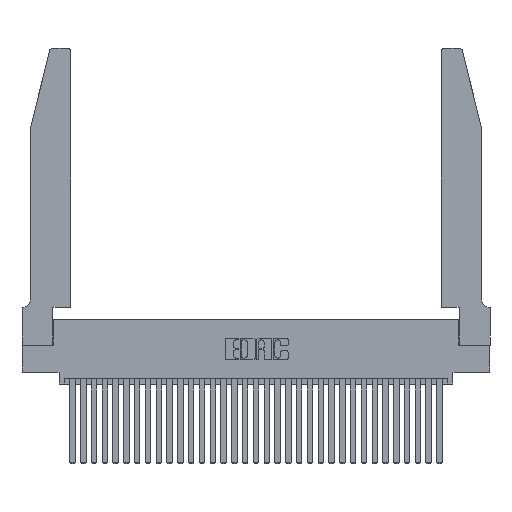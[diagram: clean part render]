
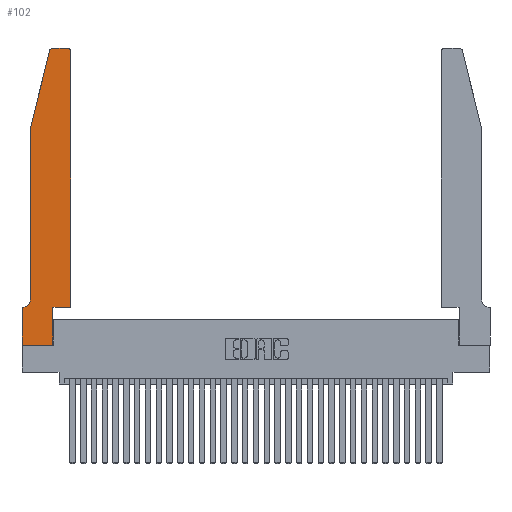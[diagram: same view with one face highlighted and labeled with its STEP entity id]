
A CAD part, top view. The second image highlights one B-rep face of the part: STEP entity #102.
In plain terms, the highlighted planar face has unit normal (0, 0, 1).
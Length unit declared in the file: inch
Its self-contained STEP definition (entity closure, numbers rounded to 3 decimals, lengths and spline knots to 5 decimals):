
#70 = CARTESIAN_POINT ( 'NONE',  ( 0., 0.35, 0.37 ) ) ;
#102 = ADVANCED_FACE ( 'NONE', ( #30458 ), #25693, .T. ) ;
#179 = CARTESIAN_POINT ( 'NONE',  ( 0.0755, 0.35, 0.37 ) ) ;
#722 = DIRECTION ( 'NONE',  ( 0., 0., 1. ) ) ;
#1178 = EDGE_CURVE ( 'NONE', #12635, #10571, #11612, .T. ) ;
#1284 = ORIENTED_EDGE ( 'NONE', *, *, #3603, .T. ) ;
#1601 = DIRECTION ( 'NONE',  ( 0., 0., 1. ) ) ;
#1818 = DIRECTION ( 'NONE',  ( 1., 0., 0. ) ) ;
#3047 = LINE ( 'NONE', #179, #16802 ) ;
#3603 = EDGE_CURVE ( 'NONE', #20287, #19433, #29973, .T. ) ;
#4251 = ORIENTED_EDGE ( 'NONE', *, *, #29277, .T. ) ;
#4355 = CARTESIAN_POINT ( 'NONE',  ( 0.4505, 0.35, 0.37 ) ) ;
#4764 = ORIENTED_EDGE ( 'NONE', *, *, #18933, .T. ) ;
#5487 = LINE ( 'NONE', #7104, #19954 ) ;
#5660 = AXIS2_PLACEMENT_3D ( 'NONE', #70, #722, #14300 ) ;
#6376 = CARTESIAN_POINT ( 'NONE',  ( 0.0055, 0.42, 0.37 ) ) ;
#7104 = CARTESIAN_POINT ( 'NONE',  ( 0., 0., 0.37 ) ) ;
#7156 = AXIS2_PLACEMENT_3D ( 'NONE', #17128, #1601, #19705 ) ;
#7888 = CARTESIAN_POINT ( 'NONE',  ( 0.4505, 0.35, 0.37 ) ) ;
#8664 = CARTESIAN_POINT ( 'NONE',  ( 0.4505, 0.35, 0.37 ) ) ;
#8717 = LINE ( 'NONE', #14898, #28163 ) ;
#8798 = CARTESIAN_POINT ( 'NONE',  ( 0.0755, 2., 0.37 ) ) ;
#8982 = DIRECTION ( 'NONE',  ( -1., 0., 0. ) ) ;
#9135 = AXIS2_PLACEMENT_3D ( 'NONE', #26910, #11807, #29425 ) ;
#9376 = VECTOR ( 'NONE', #17767, 39.37008 ) ;
#9768 = EDGE_CURVE ( 'NONE', #19433, #32056, #3047, .T. ) ;
#9842 = ORIENTED_EDGE ( 'NONE', *, *, #31726, .T. ) ;
#10044 = VERTEX_POINT ( 'NONE', #12443 ) ;
#10151 = EDGE_CURVE ( 'NONE', #27396, #27910, #31684, .T. ) ;
#10367 = DIRECTION ( 'NONE',  ( -0.239, -0.971, 0. ) ) ;
#10543 = LINE ( 'NONE', #7888, #24048 ) ;
#10571 = VERTEX_POINT ( 'NONE', #19745 ) ;
#10981 = VECTOR ( 'NONE', #30465, 39.37008 ) ;
#11612 = LINE ( 'NONE', #15123, #25077 ) ;
#11807 = DIRECTION ( 'NONE',  ( 0., 0., 1. ) ) ;
#12443 = CARTESIAN_POINT ( 'NONE',  ( 0.4505, 2.72, 0.37 ) ) ;
#12545 = CARTESIAN_POINT ( 'NONE',  ( 0., 0.35, 0.37 ) ) ;
#12607 = ORIENTED_EDGE ( 'NONE', *, *, #31337, .T. ) ;
#12635 = VERTEX_POINT ( 'NONE', #26372 ) ;
#12777 = ORIENTED_EDGE ( 'NONE', *, *, #9768, .T. ) ;
#12902 = CARTESIAN_POINT ( 'NONE',  ( 0.0755, 2., 0.37 ) ) ;
#13571 = EDGE_CURVE ( 'NONE', #24907, #10044, #10543, .T. ) ;
#14287 = ORIENTED_EDGE ( 'NONE', *, *, #1178, .T. ) ;
#14300 = DIRECTION ( 'NONE',  ( 1., 0., 0. ) ) ;
#14514 = CARTESIAN_POINT ( 'NONE',  ( 0.0055, 0.35, 0.37 ) ) ;
#14793 = DIRECTION ( 'NONE',  ( 0., -1., 0. ) ) ;
#14898 = CARTESIAN_POINT ( 'NONE',  ( 0., 0., 0.37 ) ) ;
#15123 = CARTESIAN_POINT ( 'NONE',  ( 0.2605, 2.75, 0.37 ) ) ;
#15358 = CARTESIAN_POINT ( 'NONE',  ( 0., 0., 0.37 ) ) ;
#15443 = CARTESIAN_POINT ( 'NONE',  ( 0.0755, 2., 0.37 ) ) ;
#15534 = ORIENTED_EDGE ( 'NONE', *, *, #10151, .T. ) ;
#16018 = EDGE_CURVE ( 'NONE', #32056, #17878, #5487, .T. ) ;
#16802 = VECTOR ( 'NONE', #20920, 39.37008 ) ;
#16987 = EDGE_LOOP ( 'NONE', ( #14287, #26789, #15534, #31223, #1284, #12777, #22879, #12607, #4764, #9842, #19266, #4251 ) ) ;
#17128 = CARTESIAN_POINT ( 'NONE',  ( 0.284, 2.72, 0.37 ) ) ;
#17322 = VERTEX_POINT ( 'NONE', #32947 ) ;
#17767 = DIRECTION ( 'NONE',  ( 0., 1., 0. ) ) ;
#17878 = VERTEX_POINT ( 'NONE', #15358 ) ;
#18933 = EDGE_CURVE ( 'NONE', #19783, #17322, #28796, .T. ) ;
#19266 = ORIENTED_EDGE ( 'NONE', *, *, #13571, .T. ) ;
#19433 = VERTEX_POINT ( 'NONE', #14514 ) ;
#19705 = DIRECTION ( 'NONE',  ( 1., 0., 0. ) ) ;
#19745 = CARTESIAN_POINT ( 'NONE',  ( 0.284, 2.75, 0.37 ) ) ;
#19783 = VERTEX_POINT ( 'NONE', #30955 ) ;
#19954 = VECTOR ( 'NONE', #14793, 39.37008 ) ;
#20287 = VERTEX_POINT ( 'NONE', #20462 ) ;
#20313 = CARTESIAN_POINT ( 'NONE',  ( 0.2865, 0.35, 0.37 ) ) ;
#20462 = CARTESIAN_POINT ( 'NONE',  ( 0.0755, 0.42, 0.37 ) ) ;
#20920 = DIRECTION ( 'NONE',  ( -1., 0., 0. ) ) ;
#21692 = CARTESIAN_POINT ( 'NONE',  ( 0.25487, 2.72718, 0.37 ) ) ;
#22846 = CIRCLE ( 'NONE', #9135, 0.03 ) ;
#22879 = ORIENTED_EDGE ( 'NONE', *, *, #16018, .T. ) ;
#23897 = AXIS2_PLACEMENT_3D ( 'NONE', #6376, #24228, #8982 ) ;
#23929 = DIRECTION ( 'NONE',  ( 1., 0., 0. ) ) ;
#24048 = VECTOR ( 'NONE', #25677, 39.37008 ) ;
#24228 = DIRECTION ( 'NONE',  ( 0., 0., -1. ) ) ;
#24907 = VERTEX_POINT ( 'NONE', #4355 ) ;
#25047 = VECTOR ( 'NONE', #10367, 39.37008 ) ;
#25077 = VECTOR ( 'NONE', #25166, 39.37008 ) ;
#25166 = DIRECTION ( 'NONE',  ( -1., 0., 0. ) ) ;
#25416 = VECTOR ( 'NONE', #23929, 39.37008 ) ;
#25677 = DIRECTION ( 'NONE',  ( 0., 1., 0. ) ) ;
#25693 = PLANE ( 'NONE',  #5660 ) ;
#26372 = CARTESIAN_POINT ( 'NONE',  ( 0.4205, 2.75, 0.37 ) ) ;
#26789 = ORIENTED_EDGE ( 'NONE', *, *, #27510, .T. ) ;
#26910 = CARTESIAN_POINT ( 'NONE',  ( 0.4205, 2.72, 0.37 ) ) ;
#27396 = VERTEX_POINT ( 'NONE', #21692 ) ;
#27510 = EDGE_CURVE ( 'NONE', #10571, #27396, #29155, .T. ) ;
#27910 = VERTEX_POINT ( 'NONE', #8798 ) ;
#28163 = VECTOR ( 'NONE', #1818, 39.37008 ) ;
#28308 = EDGE_CURVE ( 'NONE', #27910, #20287, #31104, .T. ) ;
#28796 = LINE ( 'NONE', #20313, #9376 ) ;
#29155 = CIRCLE ( 'NONE', #7156, 0.03 ) ;
#29277 = EDGE_CURVE ( 'NONE', #10044, #12635, #22846, .T. ) ;
#29425 = DIRECTION ( 'NONE',  ( 1., 0., 0. ) ) ;
#29973 = CIRCLE ( 'NONE', #23897, 0.07 ) ;
#30458 = FACE_OUTER_BOUND ( 'NONE', #16987, .T. ) ;
#30465 = DIRECTION ( 'NONE',  ( 0., -1., 0. ) ) ;
#30955 = CARTESIAN_POINT ( 'NONE',  ( 0.2865, 0., 0.37 ) ) ;
#31104 = LINE ( 'NONE', #12902, #10981 ) ;
#31223 = ORIENTED_EDGE ( 'NONE', *, *, #28308, .T. ) ;
#31249 = LINE ( 'NONE', #8664, #25416 ) ;
#31337 = EDGE_CURVE ( 'NONE', #17878, #19783, #8717, .T. ) ;
#31684 = LINE ( 'NONE', #15443, #25047 ) ;
#31726 = EDGE_CURVE ( 'NONE', #17322, #24907, #31249, .T. ) ;
#32056 = VERTEX_POINT ( 'NONE', #12545 ) ;
#32947 = CARTESIAN_POINT ( 'NONE',  ( 0.2865, 0.35, 0.37 ) ) ;
